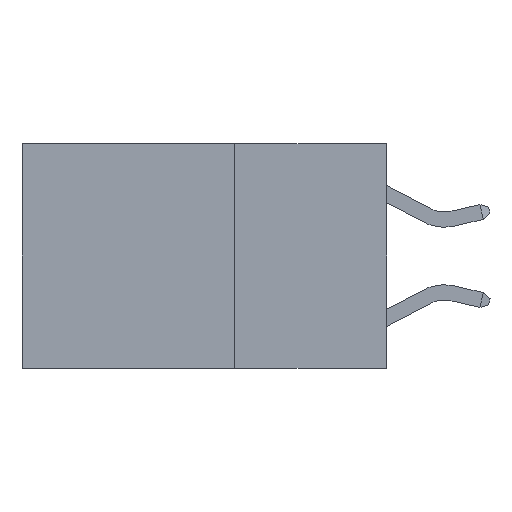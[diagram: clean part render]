
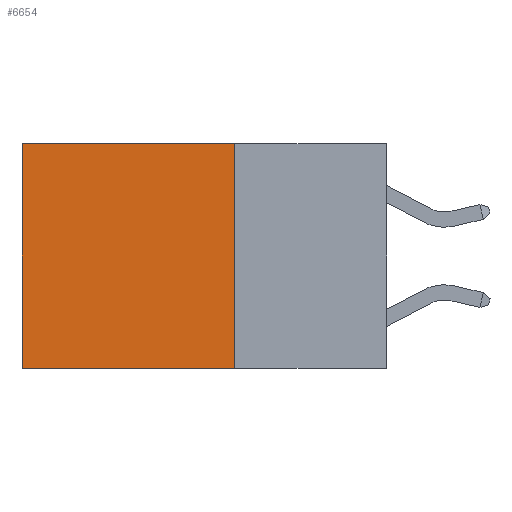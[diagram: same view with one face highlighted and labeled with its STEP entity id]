
A CAD part, left-side view. The second image highlights one B-rep face of the part: STEP entity #6654.
In plain terms, the highlighted planar face has unit normal (-1, 0, 0).
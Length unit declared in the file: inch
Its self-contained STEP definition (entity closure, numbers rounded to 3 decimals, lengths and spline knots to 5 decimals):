
#1568 = EDGE_LOOP ( 'NONE', ( #5331, #15731, #18734, #4941 ) ) ;
#2197 = DIRECTION ( 'NONE',  ( 0., 0., -1. ) ) ;
#4495 = VECTOR ( 'NONE', #27551, 39.37008 ) ;
#4941 = ORIENTED_EDGE ( 'NONE', *, *, #14671, .T. ) ;
#5331 = ORIENTED_EDGE ( 'NONE', *, *, #20502, .T. ) ;
#6103 = PLANE ( 'NONE',  #20152 ) ;
#6654 = ADVANCED_FACE ( 'NONE', ( #15211 ), #6103, .F. ) ;
#7155 = CARTESIAN_POINT ( 'NONE',  ( 0.2625, 0.6, 0. ) ) ;
#7364 = EDGE_CURVE ( 'NONE', #26128, #18466, #10088, .T. ) ;
#7845 = VECTOR ( 'NONE', #16673, 39.37008 ) ;
#8089 = LINE ( 'NONE', #20699, #4495 ) ;
#8373 = CARTESIAN_POINT ( 'NONE',  ( 0.2625, 0.6, -0.37 ) ) ;
#10088 = LINE ( 'NONE', #21006, #7845 ) ;
#12281 = CARTESIAN_POINT ( 'NONE',  ( 0.2625, 0.25, 0. ) ) ;
#13351 = VECTOR ( 'NONE', #13604, 39.37008 ) ;
#13604 = DIRECTION ( 'NONE',  ( 0., 0., -1. ) ) ;
#14671 = EDGE_CURVE ( 'NONE', #26128, #16338, #16476, .T. ) ;
#15211 = FACE_OUTER_BOUND ( 'NONE', #1568, .T. ) ;
#15731 = ORIENTED_EDGE ( 'NONE', *, *, #22527, .F. ) ;
#16338 = VERTEX_POINT ( 'NONE', #19568 ) ;
#16476 = LINE ( 'NONE', #12281, #25504 ) ;
#16673 = DIRECTION ( 'NONE',  ( 0., 0., -1. ) ) ;
#17034 = CARTESIAN_POINT ( 'NONE',  ( 0.2625, 0.25, 0. ) ) ;
#17551 = VERTEX_POINT ( 'NONE', #8373 ) ;
#18466 = VERTEX_POINT ( 'NONE', #26062 ) ;
#18734 = ORIENTED_EDGE ( 'NONE', *, *, #7364, .F. ) ;
#19358 = LINE ( 'NONE', #7155, #13351 ) ;
#19568 = CARTESIAN_POINT ( 'NONE',  ( 0.2625, 0.6, 0. ) ) ;
#20152 = AXIS2_PLACEMENT_3D ( 'NONE', #17034, #25577, #2197 ) ;
#20502 = EDGE_CURVE ( 'NONE', #16338, #17551, #19358, .T. ) ;
#20699 = CARTESIAN_POINT ( 'NONE',  ( 0.2625, 0.25, -0.37 ) ) ;
#21006 = CARTESIAN_POINT ( 'NONE',  ( 0.2625, 0.25, 0. ) ) ;
#22527 = EDGE_CURVE ( 'NONE', #18466, #17551, #8089, .T. ) ;
#23361 = CARTESIAN_POINT ( 'NONE',  ( 0.2625, 0.25, 0. ) ) ;
#25024 = DIRECTION ( 'NONE',  ( 0., 1., 0. ) ) ;
#25504 = VECTOR ( 'NONE', #25024, 39.37008 ) ;
#25577 = DIRECTION ( 'NONE',  ( 1., 0., 0. ) ) ;
#26062 = CARTESIAN_POINT ( 'NONE',  ( 0.2625, 0.25, -0.37 ) ) ;
#26128 = VERTEX_POINT ( 'NONE', #23361 ) ;
#27551 = DIRECTION ( 'NONE',  ( 0., 1., 0. ) ) ;
